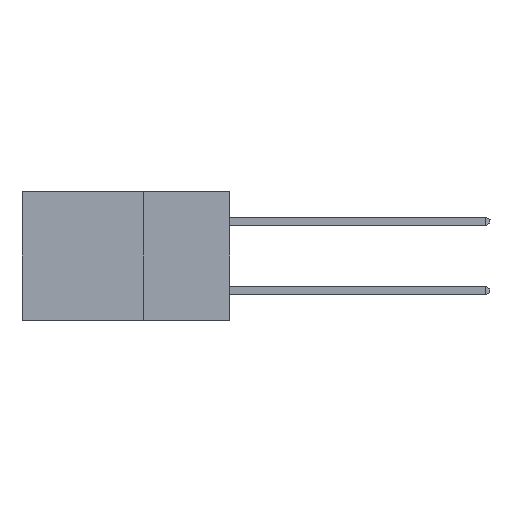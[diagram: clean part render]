
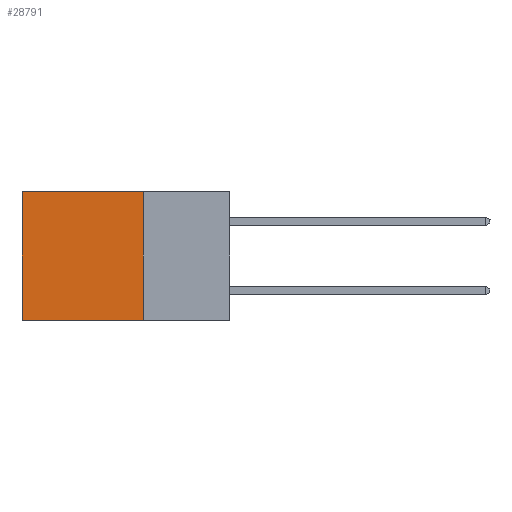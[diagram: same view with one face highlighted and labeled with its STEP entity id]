
A CAD part, left-side view. The second image highlights one B-rep face of the part: STEP entity #28791.
In plain terms, the highlighted planar face has unit normal (-1, 0, 0).
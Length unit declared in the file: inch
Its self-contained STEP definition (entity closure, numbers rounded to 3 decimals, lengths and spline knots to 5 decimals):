
#1024 = CARTESIAN_POINT ( 'NONE',  ( 0.298, 0.25, 0. ) ) ;
#2418 = EDGE_CURVE ( 'NONE', #7670, #22095, #17732, .T. ) ;
#3956 = EDGE_LOOP ( 'NONE', ( #18271, #23065, #4535, #23832 ) ) ;
#4535 = ORIENTED_EDGE ( 'NONE', *, *, #26862, .F. ) ;
#4875 = FACE_OUTER_BOUND ( 'NONE', #3956, .T. ) ;
#6134 = CARTESIAN_POINT ( 'NONE',  ( 0.298, 0.25, -0.37 ) ) ;
#6161 = PLANE ( 'NONE',  #24757 ) ;
#6173 = DIRECTION ( 'NONE',  ( 0., 1., 0. ) ) ;
#6920 = CARTESIAN_POINT ( 'NONE',  ( 0.298, 0.25, 0. ) ) ;
#7670 = VERTEX_POINT ( 'NONE', #30983 ) ;
#8715 = DIRECTION ( 'NONE',  ( 1., 0., 0. ) ) ;
#10525 = VECTOR ( 'NONE', #14386, 39.37008 ) ;
#14068 = EDGE_CURVE ( 'NONE', #15370, #22095, #29573, .T. ) ;
#14386 = DIRECTION ( 'NONE',  ( 0., 0., -1. ) ) ;
#14413 = LINE ( 'NONE', #6920, #21119 ) ;
#15370 = VERTEX_POINT ( 'NONE', #28780 ) ;
#16460 = VECTOR ( 'NONE', #30885, 39.37008 ) ;
#16962 = CARTESIAN_POINT ( 'NONE',  ( 0.298, 0.25, 0. ) ) ;
#17323 = LINE ( 'NONE', #16962, #10525 ) ;
#17732 = LINE ( 'NONE', #6134, #23515 ) ;
#18271 = ORIENTED_EDGE ( 'NONE', *, *, #14068, .T. ) ;
#18525 = CARTESIAN_POINT ( 'NONE',  ( 0.298, 0.25, 0. ) ) ;
#21119 = VECTOR ( 'NONE', #26982, 39.37008 ) ;
#22095 = VERTEX_POINT ( 'NONE', #24740 ) ;
#23065 = ORIENTED_EDGE ( 'NONE', *, *, #2418, .F. ) ;
#23515 = VECTOR ( 'NONE', #6173, 39.37008 ) ;
#23832 = ORIENTED_EDGE ( 'NONE', *, *, #25150, .T. ) ;
#24740 = CARTESIAN_POINT ( 'NONE',  ( 0.298, 0.6, -0.37 ) ) ;
#24757 = AXIS2_PLACEMENT_3D ( 'NONE', #1024, #8715, #26236 ) ;
#25150 = EDGE_CURVE ( 'NONE', #31697, #15370, #14413, .T. ) ;
#26236 = DIRECTION ( 'NONE',  ( 0., 0., -1. ) ) ;
#26862 = EDGE_CURVE ( 'NONE', #31697, #7670, #17323, .T. ) ;
#26982 = DIRECTION ( 'NONE',  ( 0., 1., 0. ) ) ;
#28528 = CARTESIAN_POINT ( 'NONE',  ( 0.298, 0.6, 0. ) ) ;
#28780 = CARTESIAN_POINT ( 'NONE',  ( 0.298, 0.6, 0. ) ) ;
#28791 = ADVANCED_FACE ( 'NONE', ( #4875 ), #6161, .F. ) ;
#29573 = LINE ( 'NONE', #28528, #16460 ) ;
#30885 = DIRECTION ( 'NONE',  ( 0., 0., -1. ) ) ;
#30983 = CARTESIAN_POINT ( 'NONE',  ( 0.298, 0.25, -0.37 ) ) ;
#31697 = VERTEX_POINT ( 'NONE', #18525 ) ;
